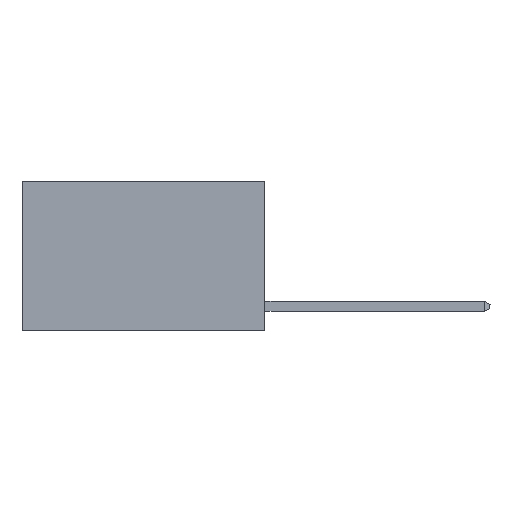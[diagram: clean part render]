
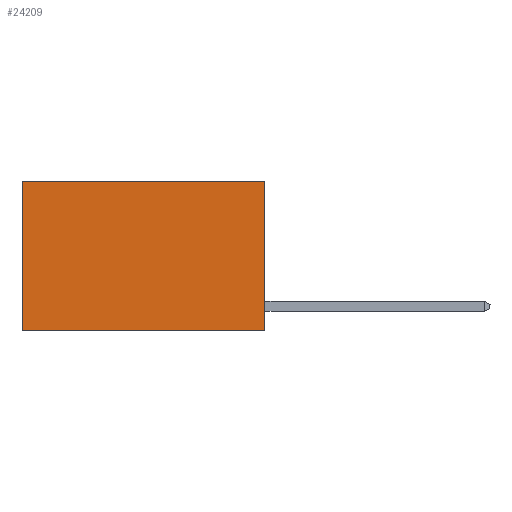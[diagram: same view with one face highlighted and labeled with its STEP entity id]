
A CAD part, left-side view. The second image highlights one B-rep face of the part: STEP entity #24209.
In plain terms, the highlighted planar face has unit normal (-1, 0, 0).
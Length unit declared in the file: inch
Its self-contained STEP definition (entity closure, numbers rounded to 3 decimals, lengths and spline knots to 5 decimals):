
#1520 = CARTESIAN_POINT ( 'NONE',  ( 0.2625, 0., 0. ) ) ;
#1791 = LINE ( 'NONE', #8966, #12508 ) ;
#1951 = VERTEX_POINT ( 'NONE', #18885 ) ;
#4781 = EDGE_CURVE ( 'NONE', #17482, #1951, #15226, .T. ) ;
#5464 = CARTESIAN_POINT ( 'NONE',  ( 0.2625, 0., -0.37 ) ) ;
#5929 = CARTESIAN_POINT ( 'NONE',  ( 0.2625, 0., 0. ) ) ;
#6208 = DIRECTION ( 'NONE',  ( 0., 0., -1. ) ) ;
#6261 = EDGE_CURVE ( 'NONE', #25549, #24441, #19933, .T. ) ;
#6630 = ORIENTED_EDGE ( 'NONE', *, *, #21504, .F. ) ;
#7039 = DIRECTION ( 'NONE',  ( 0., 1., 0. ) ) ;
#7978 = PLANE ( 'NONE',  #14693 ) ;
#8966 = CARTESIAN_POINT ( 'NONE',  ( 0.2625, 0., 0. ) ) ;
#10707 = EDGE_CURVE ( 'NONE', #24441, #1951, #12987, .T. ) ;
#10901 = DIRECTION ( 'NONE',  ( 0., 0., -1. ) ) ;
#11984 = VECTOR ( 'NONE', #24636, 39.37008 ) ;
#12349 = ORIENTED_EDGE ( 'NONE', *, *, #6261, .T. ) ;
#12508 = VECTOR ( 'NONE', #10901, 39.37008 ) ;
#12874 = VECTOR ( 'NONE', #16431, 39.37008 ) ;
#12877 = VECTOR ( 'NONE', #7039, 39.37008 ) ;
#12987 = LINE ( 'NONE', #14626, #11984 ) ;
#14626 = CARTESIAN_POINT ( 'NONE',  ( 0.2625, 0.6, 0. ) ) ;
#14648 = CARTESIAN_POINT ( 'NONE',  ( 0.2625, 0., 0. ) ) ;
#14693 = AXIS2_PLACEMENT_3D ( 'NONE', #5929, #16866, #6208 ) ;
#15226 = LINE ( 'NONE', #15565, #12877 ) ;
#15565 = CARTESIAN_POINT ( 'NONE',  ( 0.2625, 0., -0.37 ) ) ;
#15828 = ORIENTED_EDGE ( 'NONE', *, *, #10707, .T. ) ;
#16431 = DIRECTION ( 'NONE',  ( 0., 1., 0. ) ) ;
#16520 = ORIENTED_EDGE ( 'NONE', *, *, #4781, .F. ) ;
#16866 = DIRECTION ( 'NONE',  ( 1., 0., 0. ) ) ;
#17425 = CARTESIAN_POINT ( 'NONE',  ( 0.2625, 0.6, 0. ) ) ;
#17482 = VERTEX_POINT ( 'NONE', #5464 ) ;
#18885 = CARTESIAN_POINT ( 'NONE',  ( 0.2625, 0.6, -0.37 ) ) ;
#19933 = LINE ( 'NONE', #1520, #12874 ) ;
#20685 = EDGE_LOOP ( 'NONE', ( #15828, #16520, #6630, #12349 ) ) ;
#21504 = EDGE_CURVE ( 'NONE', #25549, #17482, #1791, .T. ) ;
#24209 = ADVANCED_FACE ( 'NONE', ( #27615 ), #7978, .F. ) ;
#24441 = VERTEX_POINT ( 'NONE', #17425 ) ;
#24636 = DIRECTION ( 'NONE',  ( 0., 0., -1. ) ) ;
#25549 = VERTEX_POINT ( 'NONE', #14648 ) ;
#27615 = FACE_OUTER_BOUND ( 'NONE', #20685, .T. ) ;
